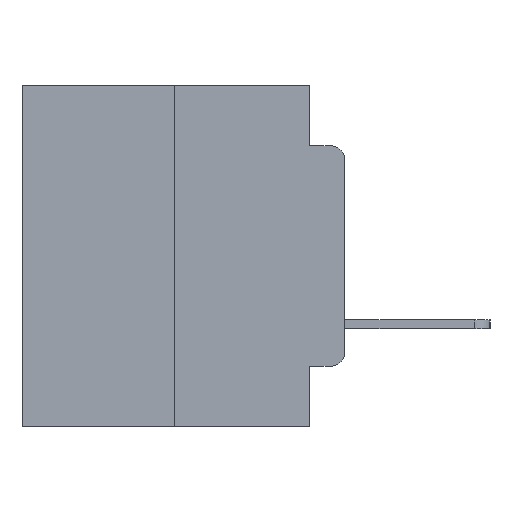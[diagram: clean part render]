
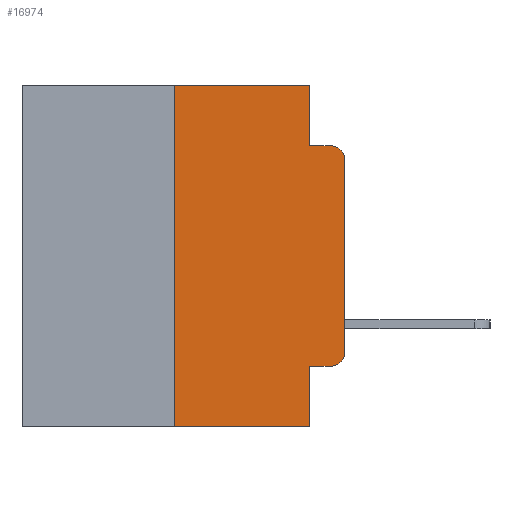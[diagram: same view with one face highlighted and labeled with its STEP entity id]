
A CAD part, left-side view. The second image highlights one B-rep face of the part: STEP entity #16974.
In plain terms, the highlighted planar face has unit normal (-1, 0, 0).
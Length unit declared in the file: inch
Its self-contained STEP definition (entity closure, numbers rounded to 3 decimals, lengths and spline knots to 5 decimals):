
#18 = VECTOR ( 'NONE', #19758, 39.37008 ) ;
#300 = LINE ( 'NONE', #17551, #10707 ) ;
#307 = FACE_OUTER_BOUND ( 'NONE', #7544, .T. ) ;
#1254 = VECTOR ( 'NONE', #5020, 39.37008 ) ;
#1625 = DIRECTION ( 'NONE',  ( 0., 0., -1. ) ) ;
#1704 = ORIENTED_EDGE ( 'NONE', *, *, #1934, .T. ) ;
#1934 = EDGE_CURVE ( 'NONE', #16446, #15884, #23423, .T. ) ;
#2428 = VECTOR ( 'NONE', #19245, 39.37008 ) ;
#2541 = EDGE_CURVE ( 'NONE', #15884, #21982, #11750, .T. ) ;
#2673 = DIRECTION ( 'NONE',  ( 0., 0., -1. ) ) ;
#2708 = EDGE_CURVE ( 'NONE', #4154, #12906, #6917, .T. ) ;
#2779 = CARTESIAN_POINT ( 'NONE',  ( 0., 0.051, 0. ) ) ;
#3261 = PLANE ( 'NONE',  #9478 ) ;
#3967 = CARTESIAN_POINT ( 'NONE',  ( 0., 0.051, -0.4115 ) ) ;
#4045 = ORIENTED_EDGE ( 'NONE', *, *, #16236, .T. ) ;
#4118 = CARTESIAN_POINT ( 'NONE',  ( 0., 0.051, -0.5 ) ) ;
#4154 = VERTEX_POINT ( 'NONE', #9493 ) ;
#5020 = DIRECTION ( 'NONE',  ( 0., -1., 0. ) ) ;
#5645 = CARTESIAN_POINT ( 'NONE',  ( 0., 0.051, -0.0885 ) ) ;
#5664 = EDGE_CURVE ( 'NONE', #22283, #8219, #300, .T. ) ;
#5745 = LINE ( 'NONE', #9430, #20054 ) ;
#6045 = ORIENTED_EDGE ( 'NONE', *, *, #21907, .F. ) ;
#6128 = DIRECTION ( 'NONE',  ( 0., -1., 0. ) ) ;
#6283 = AXIS2_PLACEMENT_3D ( 'NONE', #6666, #22102, #2673 ) ;
#6286 = VERTEX_POINT ( 'NONE', #15329 ) ;
#6666 = CARTESIAN_POINT ( 'NONE',  ( 0., 0.02, -0.3915 ) ) ;
#6917 = LINE ( 'NONE', #20643, #1254 ) ;
#7135 = EDGE_CURVE ( 'NONE', #16446, #12906, #16114, .T. ) ;
#7261 = CARTESIAN_POINT ( 'NONE',  ( 0., 0., -0.1085 ) ) ;
#7415 = CARTESIAN_POINT ( 'NONE',  ( 0., 0.25, 0. ) ) ;
#7487 = CIRCLE ( 'NONE', #9092, 0.02 ) ;
#7533 = DIRECTION ( 'NONE',  ( 0., 0., -1. ) ) ;
#7544 = EDGE_LOOP ( 'NONE', ( #4045, #14516, #15141, #20339, #10692, #6045, #16348, #11836, #1704, #22634 ) ) ;
#8219 = VERTEX_POINT ( 'NONE', #8682 ) ;
#8224 = CARTESIAN_POINT ( 'NONE',  ( 0., 0.051, 0. ) ) ;
#8237 = VECTOR ( 'NONE', #6128, 39.37008 ) ;
#8682 = CARTESIAN_POINT ( 'NONE',  ( 0., 0.051, -0.0885 ) ) ;
#9092 = AXIS2_PLACEMENT_3D ( 'NONE', #25001, #13618, #1625 ) ;
#9430 = CARTESIAN_POINT ( 'NONE',  ( 0., 0.473, 0. ) ) ;
#9478 = AXIS2_PLACEMENT_3D ( 'NONE', #17091, #19027, #7533 ) ;
#9493 = CARTESIAN_POINT ( 'NONE',  ( 0., 0.25, -0.5 ) ) ;
#9555 = LINE ( 'NONE', #12975, #19797 ) ;
#10692 = ORIENTED_EDGE ( 'NONE', *, *, #24569, .F. ) ;
#10707 = VECTOR ( 'NONE', #21449, 39.37008 ) ;
#11331 = CARTESIAN_POINT ( 'NONE',  ( 0., 0.051, -0.4115 ) ) ;
#11684 = CARTESIAN_POINT ( 'NONE',  ( 0., 0., -0.3915 ) ) ;
#11750 = CIRCLE ( 'NONE', #6283, 0.02 ) ;
#11836 = ORIENTED_EDGE ( 'NONE', *, *, #7135, .F. ) ;
#12906 = VERTEX_POINT ( 'NONE', #4118 ) ;
#12975 = CARTESIAN_POINT ( 'NONE',  ( 0., 0., 0. ) ) ;
#13618 = DIRECTION ( 'NONE',  ( -1., 0., 0. ) ) ;
#14516 = ORIENTED_EDGE ( 'NONE', *, *, #15274, .T. ) ;
#14961 = DIRECTION ( 'NONE',  ( 0., 0., 1. ) ) ;
#15141 = ORIENTED_EDGE ( 'NONE', *, *, #16482, .F. ) ;
#15274 = EDGE_CURVE ( 'NONE', #18865, #20859, #7487, .T. ) ;
#15289 = DIRECTION ( 'NONE',  ( 0., 0., 1. ) ) ;
#15329 = CARTESIAN_POINT ( 'NONE',  ( 0., 0.25, 0. ) ) ;
#15580 = CARTESIAN_POINT ( 'NONE',  ( 0., 0.02, -0.4115 ) ) ;
#15884 = VERTEX_POINT ( 'NONE', #15580 ) ;
#16114 = LINE ( 'NONE', #8224, #18 ) ;
#16236 = EDGE_CURVE ( 'NONE', #21982, #18865, #9555, .T. ) ;
#16348 = ORIENTED_EDGE ( 'NONE', *, *, #2708, .T. ) ;
#16446 = VERTEX_POINT ( 'NONE', #11331 ) ;
#16482 = EDGE_CURVE ( 'NONE', #8219, #20859, #17616, .T. ) ;
#16974 = ADVANCED_FACE ( 'NONE', ( #307 ), #3261, .F. ) ;
#17091 = CARTESIAN_POINT ( 'NONE',  ( 0., 0.473, 0. ) ) ;
#17551 = CARTESIAN_POINT ( 'NONE',  ( 0., 0.051, 0. ) ) ;
#17616 = LINE ( 'NONE', #5645, #2428 ) ;
#18865 = VERTEX_POINT ( 'NONE', #7261 ) ;
#19027 = DIRECTION ( 'NONE',  ( 1., 0., 0. ) ) ;
#19245 = DIRECTION ( 'NONE',  ( 0., -1., 0. ) ) ;
#19758 = DIRECTION ( 'NONE',  ( 0., 0., -1. ) ) ;
#19797 = VECTOR ( 'NONE', #14961, 39.37008 ) ;
#20054 = VECTOR ( 'NONE', #24521, 39.37008 ) ;
#20339 = ORIENTED_EDGE ( 'NONE', *, *, #5664, .F. ) ;
#20643 = CARTESIAN_POINT ( 'NONE',  ( 0., 0.473, -0.5 ) ) ;
#20859 = VERTEX_POINT ( 'NONE', #23691 ) ;
#21449 = DIRECTION ( 'NONE',  ( 0., 0., -1. ) ) ;
#21848 = VECTOR ( 'NONE', #15289, 39.37008 ) ;
#21907 = EDGE_CURVE ( 'NONE', #4154, #6286, #22429, .T. ) ;
#21982 = VERTEX_POINT ( 'NONE', #11684 ) ;
#22102 = DIRECTION ( 'NONE',  ( -1., 0., 0. ) ) ;
#22283 = VERTEX_POINT ( 'NONE', #2779 ) ;
#22429 = LINE ( 'NONE', #7415, #21848 ) ;
#22634 = ORIENTED_EDGE ( 'NONE', *, *, #2541, .T. ) ;
#23423 = LINE ( 'NONE', #3967, #8237 ) ;
#23691 = CARTESIAN_POINT ( 'NONE',  ( 0., 0.02, -0.0885 ) ) ;
#24521 = DIRECTION ( 'NONE',  ( 0., -1., 0. ) ) ;
#24569 = EDGE_CURVE ( 'NONE', #6286, #22283, #5745, .T. ) ;
#25001 = CARTESIAN_POINT ( 'NONE',  ( 0., 0.02, -0.1085 ) ) ;
